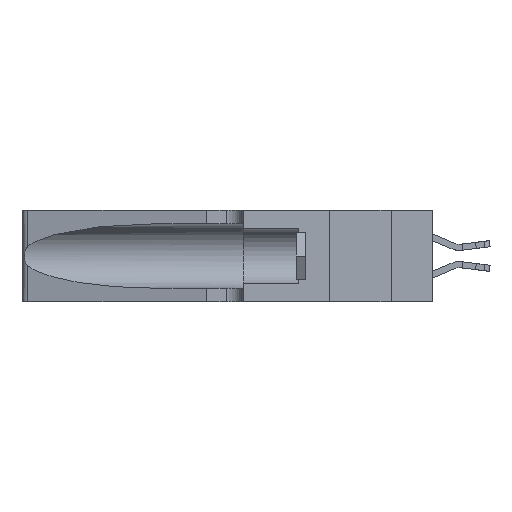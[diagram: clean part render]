
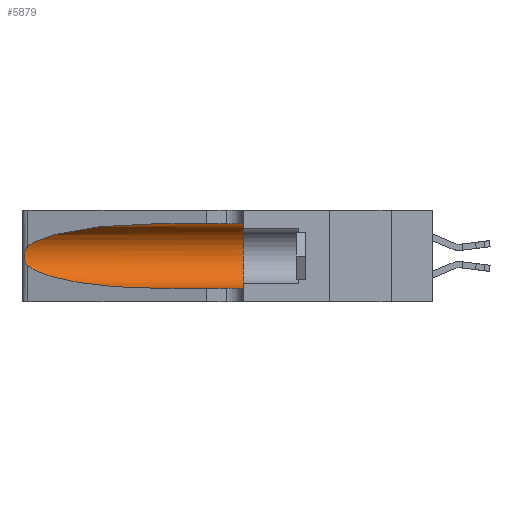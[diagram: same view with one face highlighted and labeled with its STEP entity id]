
A CAD part, left-side view. The second image highlights one B-rep face of the part: STEP entity #5879.
In plain terms, the highlighted cylindrical face has radius 3.308 mm (diameter 6.617 mm), a partial arc.
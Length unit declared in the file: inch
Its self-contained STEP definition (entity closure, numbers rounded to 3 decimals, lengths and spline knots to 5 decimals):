
#117 = LINE ( 'NONE', #17274, #24953 ) ;
#139 = DIRECTION ( 'NONE',  ( 0., -1., 0. ) ) ;
#689 = ORIENTED_EDGE ( 'NONE', *, *, #17831, .F. ) ;
#1407 = ORIENTED_EDGE ( 'NONE', *, *, #14261, .T. ) ;
#1512 =( BOUNDED_CURVE ( )  B_SPLINE_CURVE ( 3, ( #25858, #12849, #12934, #21501 ),
 .UNSPECIFIED., .F., .F. ) 
 B_SPLINE_CURVE_WITH_KNOTS ( ( 4, 4 ),
 ( 3.44316, 4.71239 ),
 .UNSPECIFIED. ) 
 CURVE ( )  GEOMETRIC_REPRESENTATION_ITEM ( )  RATIONAL_B_SPLINE_CURVE ( ( 1., 0.87, 0.87, 1. ) ) 
 REPRESENTATION_ITEM ( '' )  );
#1710 = CARTESIAN_POINT ( 'NONE',  ( 0.26018, 1.23835, 0.19895 ) ) ;
#1931 = CARTESIAN_POINT ( 'NONE',  ( 0.2373, 1.15595, 0.28018 ) ) ;
#2212 = ORIENTED_EDGE ( 'NONE', *, *, #15645, .F. ) ;
#2759 = CARTESIAN_POINT ( 'NONE',  ( 0.1305, 0.72297, 0.05475 ) ) ;
#4008 = CARTESIAN_POINT ( 'NONE',  ( 0.1305, 0.72297, 0.31525 ) ) ;
#4066 = CARTESIAN_POINT ( 'NONE',  ( 0.25856, 1.23593, 0.16098 ) ) ;
#4091 = B_SPLINE_CURVE_WITH_KNOTS ( 'NONE', 3,
 ( #7726, #26579, #22396, #16474, #18749, #1710, #20726, #6479, #14969, #4066, #17043, #6305, #24090, #22086 ),
 .UNSPECIFIED., .F., .F.,
 ( 4, 2, 2, 2, 2, 2, 4 ),
 ( 0., 0.00027, 0.00053, 0.00107, 0.0016, 0.00187, 0.00214 ),
 .UNSPECIFIED. ) ;
#5175 = CIRCLE ( 'NONE', #11602, 0.13025 ) ;
#5879 = ADVANCED_FACE ( 'NONE', ( #15494 ), #8448, .F. ) ;
#6263 = AXIS2_PLACEMENT_3D ( 'NONE', #25492, #10698, #22422 ) ;
#6305 = CARTESIAN_POINT ( 'NONE',  ( 0.25639, 1.23186, 0.15144 ) ) ;
#6479 = CARTESIAN_POINT ( 'NONE',  ( 0.26075, 1.23896, 0.178 ) ) ;
#6712 = ORIENTED_EDGE ( 'NONE', *, *, #7809, .T. ) ;
#7726 = CARTESIAN_POINT ( 'NONE',  ( 0.25487, 1.22718, 0.22369 ) ) ;
#7809 = EDGE_CURVE ( 'NONE', #13633, #26306, #117, .T. ) ;
#7841 = CARTESIAN_POINT ( 'NONE',  ( 0.1305, 0.35, 0.31525 ) ) ;
#8448 = CYLINDRICAL_SURFACE ( 'NONE', #6263, 0.13025 ) ;
#8977 = LINE ( 'NONE', #16573, #19111 ) ;
#9101 = CARTESIAN_POINT ( 'NONE',  ( 0.1305, 0.35, 0.185 ) ) ;
#10626 = DIRECTION ( 'NONE',  ( 0., 1., 0. ) ) ;
#10698 = DIRECTION ( 'NONE',  ( 0., -1., 0. ) ) ;
#11544 = CARTESIAN_POINT ( 'NONE',  ( 0.25487, 1.22718, 0.22369 ) ) ;
#11602 = AXIS2_PLACEMENT_3D ( 'NONE', #9101, #10626, #25612 ) ;
#11925 = CARTESIAN_POINT ( 'NONE',  ( 0.18966, 0.96281, 0.31525 ) ) ;
#12668 = ORIENTED_EDGE ( 'NONE', *, *, #19189, .T. ) ;
#12849 = CARTESIAN_POINT ( 'NONE',  ( 0.2373, 1.15595, 0.08982 ) ) ;
#12934 = CARTESIAN_POINT ( 'NONE',  ( 0.18966, 0.96281, 0.05475 ) ) ;
#12968 = VERTEX_POINT ( 'NONE', #7841 ) ;
#13302 = CARTESIAN_POINT ( 'NONE',  ( 0.1305, 0.35, 0.05475 ) ) ;
#13603 = EDGE_CURVE ( 'NONE', #23871, #13633, #1512, .T. ) ;
#13633 = VERTEX_POINT ( 'NONE', #2759 ) ;
#14261 = EDGE_CURVE ( 'NONE', #25278, #23871, #4091, .T. ) ;
#14969 = CARTESIAN_POINT ( 'NONE',  ( 0.26017, 1.23833, 0.17102 ) ) ;
#15291 = VERTEX_POINT ( 'NONE', #20007 ) ;
#15494 = FACE_OUTER_BOUND ( 'NONE', #27499, .T. ) ;
#15645 = EDGE_CURVE ( 'NONE', #15291, #12968, #8977, .T. ) ;
#16474 = CARTESIAN_POINT ( 'NONE',  ( 0.25787, 1.23484, 0.2124 ) ) ;
#16573 = CARTESIAN_POINT ( 'NONE',  ( 0.1305, 1.61858, 0.31525 ) ) ;
#17020 =( BOUNDED_CURVE ( )  B_SPLINE_CURVE ( 3, ( #4008, #11925, #1931, #18288 ),
 .UNSPECIFIED., .F., .T. ) 
 B_SPLINE_CURVE_WITH_KNOTS ( ( 4, 4 ),
 ( 1.5708, 2.84003 ),
 .UNSPECIFIED. ) 
 CURVE ( )  GEOMETRIC_REPRESENTATION_ITEM ( )  RATIONAL_B_SPLINE_CURVE ( ( 1., 0.87, 0.87, 1. ) ) 
 REPRESENTATION_ITEM ( '' )  );
#17043 = CARTESIAN_POINT ( 'NONE',  ( 0.25789, 1.23486, 0.15765 ) ) ;
#17274 = CARTESIAN_POINT ( 'NONE',  ( 0.1305, 1.61858, 0.05475 ) ) ;
#17831 = EDGE_CURVE ( 'NONE', #12968, #26306, #5175, .T. ) ;
#18288 = CARTESIAN_POINT ( 'NONE',  ( 0.25487, 1.22718, 0.22369 ) ) ;
#18749 = CARTESIAN_POINT ( 'NONE',  ( 0.25854, 1.2359, 0.20912 ) ) ;
#19111 = VECTOR ( 'NONE', #25247, 39.37008 ) ;
#19189 = EDGE_CURVE ( 'NONE', #15291, #25278, #17020, .T. ) ;
#20007 = CARTESIAN_POINT ( 'NONE',  ( 0.1305, 0.72297, 0.31525 ) ) ;
#20684 = CARTESIAN_POINT ( 'NONE',  ( 0.25487, 1.22718, 0.14631 ) ) ;
#20726 = CARTESIAN_POINT ( 'NONE',  ( 0.26075, 1.23896, 0.19203 ) ) ;
#21501 = CARTESIAN_POINT ( 'NONE',  ( 0.1305, 0.72297, 0.05475 ) ) ;
#22086 = CARTESIAN_POINT ( 'NONE',  ( 0.25487, 1.22718, 0.14631 ) ) ;
#22396 = CARTESIAN_POINT ( 'NONE',  ( 0.25639, 1.23184, 0.21858 ) ) ;
#22422 = DIRECTION ( 'NONE',  ( 0., 0., -1. ) ) ;
#23871 = VERTEX_POINT ( 'NONE', #20684 ) ;
#24090 = CARTESIAN_POINT ( 'NONE',  ( 0.25555, 1.22993, 0.14849 ) ) ;
#24953 = VECTOR ( 'NONE', #139, 39.37008 ) ;
#25247 = DIRECTION ( 'NONE',  ( 0., -1., 0. ) ) ;
#25278 = VERTEX_POINT ( 'NONE', #11544 ) ;
#25492 = CARTESIAN_POINT ( 'NONE',  ( 0.1305, 1.61858, 0.185 ) ) ;
#25499 = ORIENTED_EDGE ( 'NONE', *, *, #13603, .T. ) ;
#25612 = DIRECTION ( 'NONE',  ( 0., 0., 1. ) ) ;
#25858 = CARTESIAN_POINT ( 'NONE',  ( 0.25487, 1.22718, 0.14631 ) ) ;
#26306 = VERTEX_POINT ( 'NONE', #13302 ) ;
#26579 = CARTESIAN_POINT ( 'NONE',  ( 0.25555, 1.22994, 0.2215 ) ) ;
#27499 = EDGE_LOOP ( 'NONE', ( #12668, #1407, #25499, #6712, #689, #2212 ) ) ;
